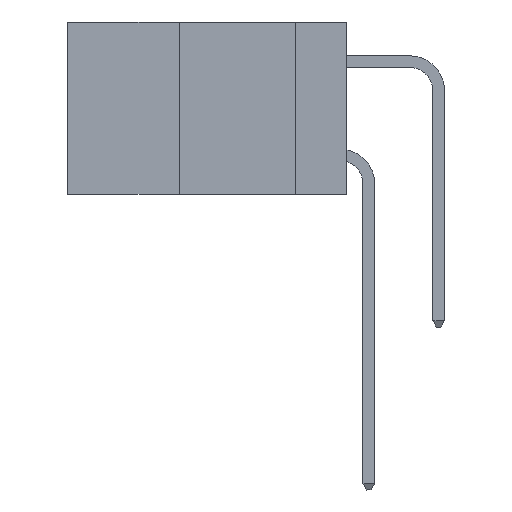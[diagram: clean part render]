
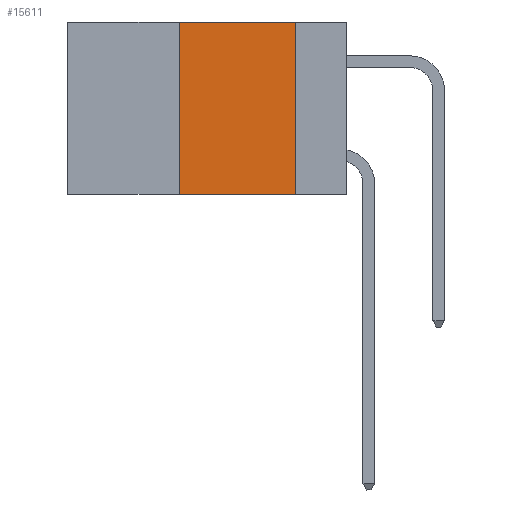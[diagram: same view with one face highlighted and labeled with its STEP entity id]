
A CAD part, left-side view. The second image highlights one B-rep face of the part: STEP entity #15611.
In plain terms, the highlighted planar face has unit normal (-1, 0, 0).
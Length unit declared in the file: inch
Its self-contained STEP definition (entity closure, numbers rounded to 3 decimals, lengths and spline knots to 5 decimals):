
#396 = DIRECTION ( 'NONE',  ( 1., 0., 0. ) ) ;
#2054 = VERTEX_POINT ( 'NONE', #8929 ) ;
#2274 = EDGE_CURVE ( 'NONE', #2991, #10257, #2302, .T. ) ;
#2302 = LINE ( 'NONE', #17336, #20882 ) ;
#2991 = VERTEX_POINT ( 'NONE', #5169 ) ;
#3110 = ORIENTED_EDGE ( 'NONE', *, *, #23143, .T. ) ;
#3166 = VECTOR ( 'NONE', #10476, 39.37008 ) ;
#3855 = FACE_OUTER_BOUND ( 'NONE', #6753, .T. ) ;
#4500 = CARTESIAN_POINT ( 'NONE',  ( 0., 0.11, 0. ) ) ;
#5169 = CARTESIAN_POINT ( 'NONE',  ( 0., 0.36, 0. ) ) ;
#5870 = EDGE_CURVE ( 'NONE', #2054, #2991, #18025, .T. ) ;
#6105 = DIRECTION ( 'NONE',  ( 0., 0., 1. ) ) ;
#6753 = EDGE_LOOP ( 'NONE', ( #7954, #8610, #26912, #3110 ) ) ;
#6777 = PLANE ( 'NONE',  #10181 ) ;
#7653 = LINE ( 'NONE', #13182, #12575 ) ;
#7954 = ORIENTED_EDGE ( 'NONE', *, *, #25034, .F. ) ;
#8610 = ORIENTED_EDGE ( 'NONE', *, *, #2274, .F. ) ;
#8929 = CARTESIAN_POINT ( 'NONE',  ( 0., 0.36, -0.37 ) ) ;
#10181 = AXIS2_PLACEMENT_3D ( 'NONE', #16992, #396, #13028 ) ;
#10257 = VERTEX_POINT ( 'NONE', #4500 ) ;
#10476 = DIRECTION ( 'NONE',  ( 0., 0., -1. ) ) ;
#12515 = VECTOR ( 'NONE', #6105, 39.37008 ) ;
#12575 = VECTOR ( 'NONE', #23510, 39.37008 ) ;
#13028 = DIRECTION ( 'NONE',  ( 0., 0., -1. ) ) ;
#13182 = CARTESIAN_POINT ( 'NONE',  ( 0., 0.6, -0.37 ) ) ;
#15589 = VERTEX_POINT ( 'NONE', #23255 ) ;
#15611 = ADVANCED_FACE ( 'NONE', ( #3855 ), #6777, .F. ) ;
#16964 = CARTESIAN_POINT ( 'NONE',  ( 0., 0.11, 0. ) ) ;
#16992 = CARTESIAN_POINT ( 'NONE',  ( 0., 0.6, 0. ) ) ;
#17336 = CARTESIAN_POINT ( 'NONE',  ( 0., 0.6, 0. ) ) ;
#18025 = LINE ( 'NONE', #25107, #12515 ) ;
#20871 = DIRECTION ( 'NONE',  ( 0., -1., 0. ) ) ;
#20882 = VECTOR ( 'NONE', #20871, 39.37008 ) ;
#21730 = LINE ( 'NONE', #16964, #3166 ) ;
#23143 = EDGE_CURVE ( 'NONE', #2054, #15589, #7653, .T. ) ;
#23255 = CARTESIAN_POINT ( 'NONE',  ( 0., 0.11, -0.37 ) ) ;
#23510 = DIRECTION ( 'NONE',  ( 0., -1., 0. ) ) ;
#25034 = EDGE_CURVE ( 'NONE', #10257, #15589, #21730, .T. ) ;
#25107 = CARTESIAN_POINT ( 'NONE',  ( 0., 0.36, 0. ) ) ;
#26912 = ORIENTED_EDGE ( 'NONE', *, *, #5870, .F. ) ;
